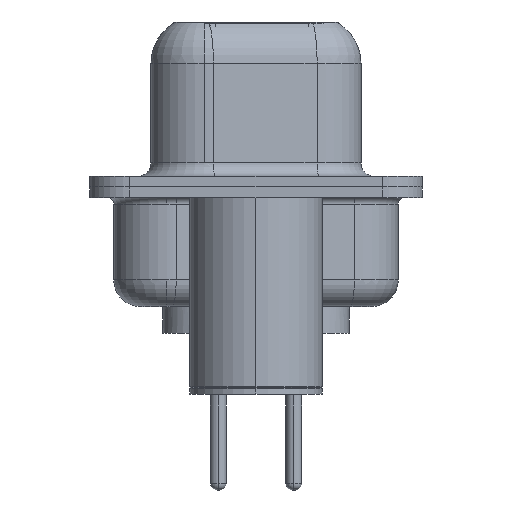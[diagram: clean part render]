
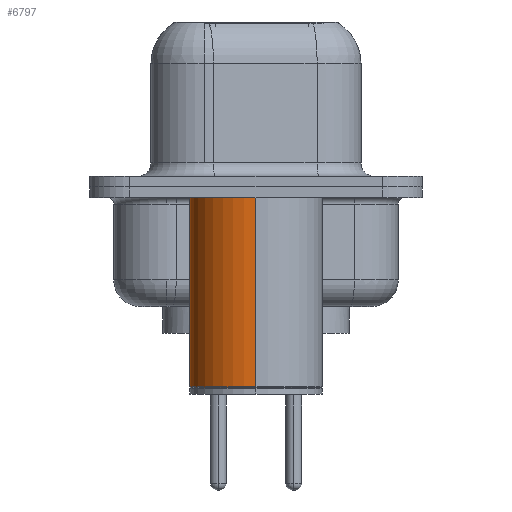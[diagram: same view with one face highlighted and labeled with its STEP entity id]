
A CAD part, left-side view. The second image highlights one B-rep face of the part: STEP entity #6797.
In plain terms, the highlighted cylindrical face has radius 2.5 mm (diameter 5 mm), a partial arc.
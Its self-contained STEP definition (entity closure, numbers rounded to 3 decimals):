
#901 = CARTESIAN_POINT ( 'NONE',  ( 2.5, 0., -0.4 ) ) ;
#1024 = CIRCLE ( 'NONE', #1906, 2.5 ) ;
#1037 = DIRECTION ( 'NONE',  ( 0., 0., 1. ) ) ;
#1544 = VERTEX_POINT ( 'NONE', #4505 ) ;
#1906 = AXIS2_PLACEMENT_3D ( 'NONE', #8049, #1037, #9542 ) ;
#1989 = EDGE_LOOP ( 'NONE', ( #17887, #6574, #14039, #3385 ) ) ;
#2369 = DIRECTION ( 'NONE',  ( 1., 0., 0. ) ) ;
#2600 = VERTEX_POINT ( 'NONE', #15282 ) ;
#2889 = DIRECTION ( 'NONE',  ( 0., 0., 1. ) ) ;
#2968 = AXIS2_PLACEMENT_3D ( 'NONE', #12509, #15314, #9428 ) ;
#3167 = CIRCLE ( 'NONE', #18417, 2.5 ) ;
#3385 = ORIENTED_EDGE ( 'NONE', *, *, #5329, .F. ) ;
#3682 = DIRECTION ( 'NONE',  ( 0., 0., 1. ) ) ;
#4505 = CARTESIAN_POINT ( 'NONE',  ( -2.5, 0., -7.525 ) ) ;
#4737 = LINE ( 'NONE', #4824, #8808 ) ;
#4824 = CARTESIAN_POINT ( 'NONE',  ( 2.5, 0., 0.581 ) ) ;
#5329 = EDGE_CURVE ( 'NONE', #2600, #5387, #4737, .T. ) ;
#5387 = VERTEX_POINT ( 'NONE', #901 ) ;
#5607 = LINE ( 'NONE', #11318, #18504 ) ;
#6574 = ORIENTED_EDGE ( 'NONE', *, *, #6619, .T. ) ;
#6619 = EDGE_CURVE ( 'NONE', #1544, #9104, #5607, .T. ) ;
#6797 = ADVANCED_FACE ( 'NONE', ( #10932 ), #14021, .T. ) ;
#8049 = CARTESIAN_POINT ( 'NONE',  ( 0., 0., -7.525 ) ) ;
#8808 = VECTOR ( 'NONE', #10548, 1000. ) ;
#9104 = VERTEX_POINT ( 'NONE', #15854 ) ;
#9428 = DIRECTION ( 'NONE',  ( 1., 0., 0. ) ) ;
#9542 = DIRECTION ( 'NONE',  ( 1., 0., 0. ) ) ;
#10548 = DIRECTION ( 'NONE',  ( 0., 0., 1. ) ) ;
#10932 = FACE_OUTER_BOUND ( 'NONE', #1989, .T. ) ;
#11318 = CARTESIAN_POINT ( 'NONE',  ( -2.5, 0., 0.581 ) ) ;
#12006 = CARTESIAN_POINT ( 'NONE',  ( 0., 0., -0.4 ) ) ;
#12509 = CARTESIAN_POINT ( 'NONE',  ( 0., 0., 0.581 ) ) ;
#13300 = EDGE_CURVE ( 'NONE', #2600, #1544, #1024, .T. ) ;
#14021 = CYLINDRICAL_SURFACE ( 'NONE', #2968, 2.5 ) ;
#14039 = ORIENTED_EDGE ( 'NONE', *, *, #16778, .F. ) ;
#15282 = CARTESIAN_POINT ( 'NONE',  ( 2.5, 0., -7.525 ) ) ;
#15314 = DIRECTION ( 'NONE',  ( 0., 0., 1. ) ) ;
#15854 = CARTESIAN_POINT ( 'NONE',  ( -2.5, 0., -0.4 ) ) ;
#16778 = EDGE_CURVE ( 'NONE', #5387, #9104, #3167, .T. ) ;
#17887 = ORIENTED_EDGE ( 'NONE', *, *, #13300, .T. ) ;
#18417 = AXIS2_PLACEMENT_3D ( 'NONE', #12006, #3682, #2369 ) ;
#18504 = VECTOR ( 'NONE', #2889, 1000. ) ;
